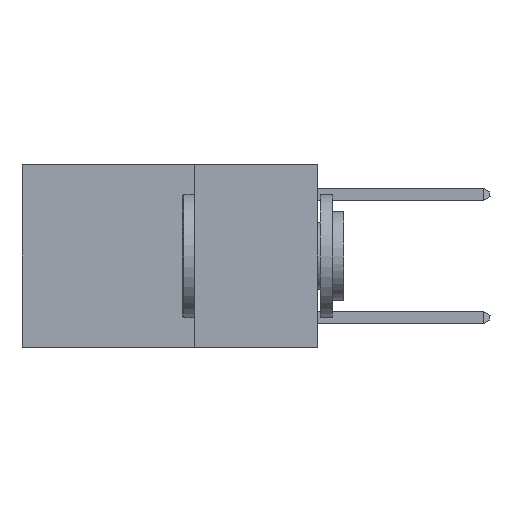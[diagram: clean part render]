
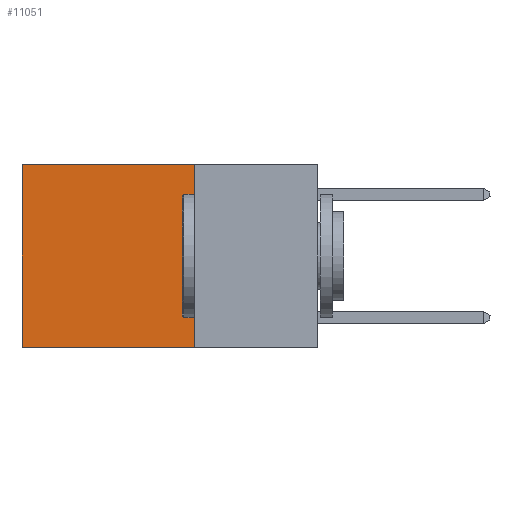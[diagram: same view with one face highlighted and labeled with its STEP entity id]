
A CAD part, left-side view. The second image highlights one B-rep face of the part: STEP entity #11051.
In plain terms, the highlighted planar face has unit normal (-1, 0, 0).
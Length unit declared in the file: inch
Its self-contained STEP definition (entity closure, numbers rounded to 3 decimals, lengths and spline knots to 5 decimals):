
#1245 = VECTOR ( 'NONE', #4375, 39.37008 ) ;
#1529 = LINE ( 'NONE', #4358, #6443 ) ;
#1541 = ORIENTED_EDGE ( 'NONE', *, *, #12451, .F. ) ;
#1698 = FACE_OUTER_BOUND ( 'NONE', #2407, .T. ) ;
#2407 = EDGE_LOOP ( 'NONE', ( #5905, #1541, #7786, #7245 ) ) ;
#2569 = CARTESIAN_POINT ( 'NONE',  ( 0.2625, 0.25, -0.37 ) ) ;
#2700 = EDGE_CURVE ( 'NONE', #6278, #12170, #1529, .T. ) ;
#2771 = VECTOR ( 'NONE', #5547, 39.37008 ) ;
#2773 = EDGE_CURVE ( 'NONE', #3220, #11563, #3716, .T. ) ;
#3220 = VERTEX_POINT ( 'NONE', #6099 ) ;
#3586 = DIRECTION ( 'NONE',  ( 0., 1., 0. ) ) ;
#3716 = LINE ( 'NONE', #7630, #2771 ) ;
#3769 = DIRECTION ( 'NONE',  ( 1., 0., 0. ) ) ;
#4014 = CARTESIAN_POINT ( 'NONE',  ( 0.2625, 0.25, 0. ) ) ;
#4358 = CARTESIAN_POINT ( 'NONE',  ( 0.2625, 0.25, 0. ) ) ;
#4375 = DIRECTION ( 'NONE',  ( 0., 1., 0. ) ) ;
#4415 = DIRECTION ( 'NONE',  ( 0., 0., -1. ) ) ;
#4559 = AXIS2_PLACEMENT_3D ( 'NONE', #4991, #3769, #12426 ) ;
#4991 = CARTESIAN_POINT ( 'NONE',  ( 0.2625, 0.25, 0. ) ) ;
#5547 = DIRECTION ( 'NONE',  ( 0., 0., -1. ) ) ;
#5594 = PLANE ( 'NONE',  #4559 ) ;
#5905 = ORIENTED_EDGE ( 'NONE', *, *, #2773, .T. ) ;
#6099 = CARTESIAN_POINT ( 'NONE',  ( 0.2625, 0.6, 0. ) ) ;
#6278 = VERTEX_POINT ( 'NONE', #4014 ) ;
#6443 = VECTOR ( 'NONE', #4415, 39.37008 ) ;
#6495 = LINE ( 'NONE', #2569, #9919 ) ;
#7245 = ORIENTED_EDGE ( 'NONE', *, *, #8387, .T. ) ;
#7630 = CARTESIAN_POINT ( 'NONE',  ( 0.2625, 0.6, 0. ) ) ;
#7786 = ORIENTED_EDGE ( 'NONE', *, *, #2700, .F. ) ;
#8387 = EDGE_CURVE ( 'NONE', #6278, #3220, #11214, .T. ) ;
#9108 = CARTESIAN_POINT ( 'NONE',  ( 0.2625, 0.25, 0. ) ) ;
#9919 = VECTOR ( 'NONE', #3586, 39.37008 ) ;
#11051 = ADVANCED_FACE ( 'NONE', ( #1698 ), #5594, .F. ) ;
#11214 = LINE ( 'NONE', #9108, #1245 ) ;
#11563 = VERTEX_POINT ( 'NONE', #12006 ) ;
#12006 = CARTESIAN_POINT ( 'NONE',  ( 0.2625, 0.6, -0.37 ) ) ;
#12170 = VERTEX_POINT ( 'NONE', #12354 ) ;
#12354 = CARTESIAN_POINT ( 'NONE',  ( 0.2625, 0.25, -0.37 ) ) ;
#12426 = DIRECTION ( 'NONE',  ( 0., 0., -1. ) ) ;
#12451 = EDGE_CURVE ( 'NONE', #12170, #11563, #6495, .T. ) ;
